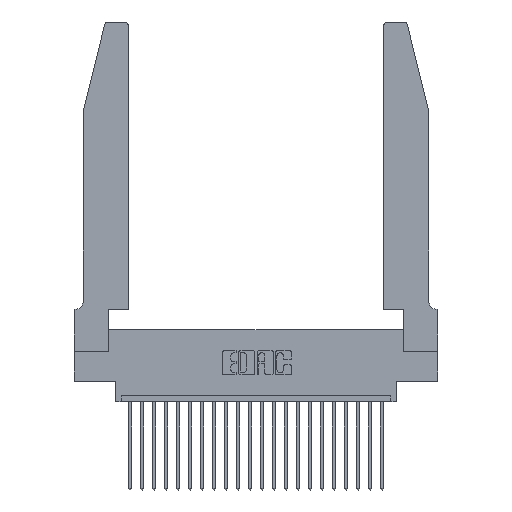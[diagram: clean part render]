
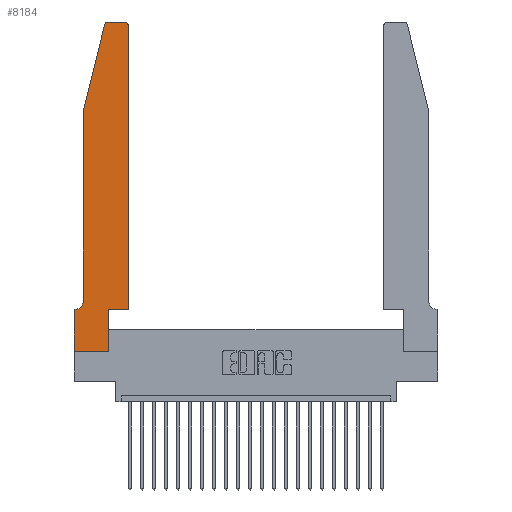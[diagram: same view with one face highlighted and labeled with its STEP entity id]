
A CAD part, top view. The second image highlights one B-rep face of the part: STEP entity #8184.
In plain terms, the highlighted planar face has unit normal (0, 0, 1).
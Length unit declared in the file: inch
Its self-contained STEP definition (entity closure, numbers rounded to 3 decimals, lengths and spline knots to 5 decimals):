
#109 = CARTESIAN_POINT ( 'NONE',  ( 0.2865, 0.35, 0.37 ) ) ;
#598 = EDGE_CURVE ( 'NONE', #17308, #19172, #11989, .T. ) ;
#650 = VERTEX_POINT ( 'NONE', #14149 ) ;
#703 = VERTEX_POINT ( 'NONE', #23837 ) ;
#859 = CIRCLE ( 'NONE', #17976, 0.07 ) ;
#952 = DIRECTION ( 'NONE',  ( 1., 0., 0. ) ) ;
#1212 = CIRCLE ( 'NONE', #1248, 0.03 ) ;
#1248 = AXIS2_PLACEMENT_3D ( 'NONE', #2841, #13752, #952 ) ;
#1768 = VECTOR ( 'NONE', #14053, 39.37008 ) ;
#2087 = VECTOR ( 'NONE', #8701, 39.37008 ) ;
#2097 = VERTEX_POINT ( 'NONE', #2814 ) ;
#2108 = EDGE_CURVE ( 'NONE', #703, #19075, #14290, .T. ) ;
#2349 = EDGE_LOOP ( 'NONE', ( #12403, #5897, #7508, #18850, #12496, #13695, #18003, #14114, #16219, #9245, #10420, #18735 ) ) ;
#2814 = CARTESIAN_POINT ( 'NONE',  ( 0.0755, 2., 0.37 ) ) ;
#2841 = CARTESIAN_POINT ( 'NONE',  ( 0.284, 2.72, 0.37 ) ) ;
#2908 = LINE ( 'NONE', #17880, #7589 ) ;
#3361 = PLANE ( 'NONE',  #5012 ) ;
#4660 = CARTESIAN_POINT ( 'NONE',  ( 0., 0., 0.37 ) ) ;
#5012 = AXIS2_PLACEMENT_3D ( 'NONE', #11074, #5936, #11238 ) ;
#5088 = CARTESIAN_POINT ( 'NONE',  ( 0.284, 2.75, 0.37 ) ) ;
#5367 = EDGE_CURVE ( 'NONE', #19075, #13464, #1212, .T. ) ;
#5378 = CARTESIAN_POINT ( 'NONE',  ( 0.0755, 0.35, 0.37 ) ) ;
#5440 = DIRECTION ( 'NONE',  ( 1., 0., 0. ) ) ;
#5493 = VECTOR ( 'NONE', #7453, 39.37008 ) ;
#5654 = CARTESIAN_POINT ( 'NONE',  ( 0.0055, 0.42, 0.37 ) ) ;
#5675 = CARTESIAN_POINT ( 'NONE',  ( 0.2865, 0.35, 0.37 ) ) ;
#5897 = ORIENTED_EDGE ( 'NONE', *, *, #5367, .T. ) ;
#5936 = DIRECTION ( 'NONE',  ( 0., 0., 1. ) ) ;
#6079 = VECTOR ( 'NONE', #14613, 39.37008 ) ;
#6098 = LINE ( 'NONE', #109, #5493 ) ;
#6214 = VERTEX_POINT ( 'NONE', #5675 ) ;
#6415 = AXIS2_PLACEMENT_3D ( 'NONE', #22084, #14676, #5440 ) ;
#6576 = VECTOR ( 'NONE', #17098, 39.37008 ) ;
#6652 = CARTESIAN_POINT ( 'NONE',  ( 0.0055, 0.35, 0.37 ) ) ;
#6658 = CARTESIAN_POINT ( 'NONE',  ( 0., 0., 0.37 ) ) ;
#6932 = LINE ( 'NONE', #5378, #6079 ) ;
#6971 = CARTESIAN_POINT ( 'NONE',  ( 0.0755, 0.42, 0.37 ) ) ;
#7022 = EDGE_CURVE ( 'NONE', #15089, #13317, #2908, .T. ) ;
#7386 = EDGE_CURVE ( 'NONE', #13317, #703, #19847, .T. ) ;
#7453 = DIRECTION ( 'NONE',  ( 0., 1., 0. ) ) ;
#7508 = ORIENTED_EDGE ( 'NONE', *, *, #22307, .T. ) ;
#7589 = VECTOR ( 'NONE', #21375, 39.37008 ) ;
#7786 = DIRECTION ( 'NONE',  ( -0.239, -0.971, 0. ) ) ;
#8049 = LINE ( 'NONE', #22616, #6576 ) ;
#8184 = ADVANCED_FACE ( 'NONE', ( #10406 ), #3361, .T. ) ;
#8701 = DIRECTION ( 'NONE',  ( 1., 0., 0. ) ) ;
#9245 = ORIENTED_EDGE ( 'NONE', *, *, #10202, .T. ) ;
#10202 = EDGE_CURVE ( 'NONE', #6214, #15089, #21714, .T. ) ;
#10406 = FACE_OUTER_BOUND ( 'NONE', #2349, .T. ) ;
#10420 = ORIENTED_EDGE ( 'NONE', *, *, #7022, .T. ) ;
#10716 = CARTESIAN_POINT ( 'NONE',  ( 0.25487, 2.72718, 0.37 ) ) ;
#10890 = VERTEX_POINT ( 'NONE', #6652 ) ;
#11074 = CARTESIAN_POINT ( 'NONE',  ( 0., 0.35, 0.37 ) ) ;
#11238 = DIRECTION ( 'NONE',  ( 1., 0., 0. ) ) ;
#11373 = DIRECTION ( 'NONE',  ( -1., 0., 0. ) ) ;
#11989 = LINE ( 'NONE', #6658, #2087 ) ;
#12030 = CARTESIAN_POINT ( 'NONE',  ( 0.4505, 2.72, 0.37 ) ) ;
#12403 = ORIENTED_EDGE ( 'NONE', *, *, #2108, .T. ) ;
#12496 = ORIENTED_EDGE ( 'NONE', *, *, #23728, .T. ) ;
#12852 = VECTOR ( 'NONE', #7786, 39.37008 ) ;
#13232 = DIRECTION ( 'NONE',  ( 1., 0., 0. ) ) ;
#13317 = VERTEX_POINT ( 'NONE', #12030 ) ;
#13464 = VERTEX_POINT ( 'NONE', #10716 ) ;
#13695 = ORIENTED_EDGE ( 'NONE', *, *, #15535, .T. ) ;
#13752 = DIRECTION ( 'NONE',  ( 0., 0., 1. ) ) ;
#13868 = DIRECTION ( 'NONE',  ( 0., -1., 0. ) ) ;
#14053 = DIRECTION ( 'NONE',  ( -1., 0., 0. ) ) ;
#14114 = ORIENTED_EDGE ( 'NONE', *, *, #598, .T. ) ;
#14149 = CARTESIAN_POINT ( 'NONE',  ( 0., 0.35, 0.37 ) ) ;
#14290 = LINE ( 'NONE', #19969, #1768 ) ;
#14404 = VECTOR ( 'NONE', #13868, 39.37008 ) ;
#14557 = CARTESIAN_POINT ( 'NONE',  ( 0.2865, 0., 0.37 ) ) ;
#14613 = DIRECTION ( 'NONE',  ( -1., 0., 0. ) ) ;
#14676 = DIRECTION ( 'NONE',  ( 0., 0., 1. ) ) ;
#15089 = VERTEX_POINT ( 'NONE', #18897 ) ;
#15121 = EDGE_CURVE ( 'NONE', #19172, #6214, #6098, .T. ) ;
#15535 = EDGE_CURVE ( 'NONE', #10890, #650, #6932, .T. ) ;
#16219 = ORIENTED_EDGE ( 'NONE', *, *, #15121, .T. ) ;
#17085 = CARTESIAN_POINT ( 'NONE',  ( 0.4505, 0.35, 0.37 ) ) ;
#17098 = DIRECTION ( 'NONE',  ( 0., -1., 0. ) ) ;
#17258 = LINE ( 'NONE', #22768, #12852 ) ;
#17308 = VERTEX_POINT ( 'NONE', #22420 ) ;
#17502 = EDGE_CURVE ( 'NONE', #2097, #20253, #8049, .T. ) ;
#17880 = CARTESIAN_POINT ( 'NONE',  ( 0.4505, 0.35, 0.37 ) ) ;
#17932 = VECTOR ( 'NONE', #13232, 39.37008 ) ;
#17976 = AXIS2_PLACEMENT_3D ( 'NONE', #5654, #22532, #11373 ) ;
#18003 = ORIENTED_EDGE ( 'NONE', *, *, #20797, .T. ) ;
#18735 = ORIENTED_EDGE ( 'NONE', *, *, #7386, .T. ) ;
#18850 = ORIENTED_EDGE ( 'NONE', *, *, #17502, .T. ) ;
#18897 = CARTESIAN_POINT ( 'NONE',  ( 0.4505, 0.35, 0.37 ) ) ;
#19075 = VERTEX_POINT ( 'NONE', #5088 ) ;
#19172 = VERTEX_POINT ( 'NONE', #14557 ) ;
#19399 = LINE ( 'NONE', #4660, #14404 ) ;
#19847 = CIRCLE ( 'NONE', #6415, 0.03 ) ;
#19969 = CARTESIAN_POINT ( 'NONE',  ( 0.2605, 2.75, 0.37 ) ) ;
#20253 = VERTEX_POINT ( 'NONE', #6971 ) ;
#20797 = EDGE_CURVE ( 'NONE', #650, #17308, #19399, .T. ) ;
#21375 = DIRECTION ( 'NONE',  ( 0., 1., 0. ) ) ;
#21714 = LINE ( 'NONE', #17085, #17932 ) ;
#22084 = CARTESIAN_POINT ( 'NONE',  ( 0.4205, 2.72, 0.37 ) ) ;
#22307 = EDGE_CURVE ( 'NONE', #13464, #2097, #17258, .T. ) ;
#22420 = CARTESIAN_POINT ( 'NONE',  ( 0., 0., 0.37 ) ) ;
#22532 = DIRECTION ( 'NONE',  ( 0., 0., -1. ) ) ;
#22616 = CARTESIAN_POINT ( 'NONE',  ( 0.0755, 2., 0.37 ) ) ;
#22768 = CARTESIAN_POINT ( 'NONE',  ( 0.0755, 2., 0.37 ) ) ;
#23728 = EDGE_CURVE ( 'NONE', #20253, #10890, #859, .T. ) ;
#23837 = CARTESIAN_POINT ( 'NONE',  ( 0.4205, 2.75, 0.37 ) ) ;
